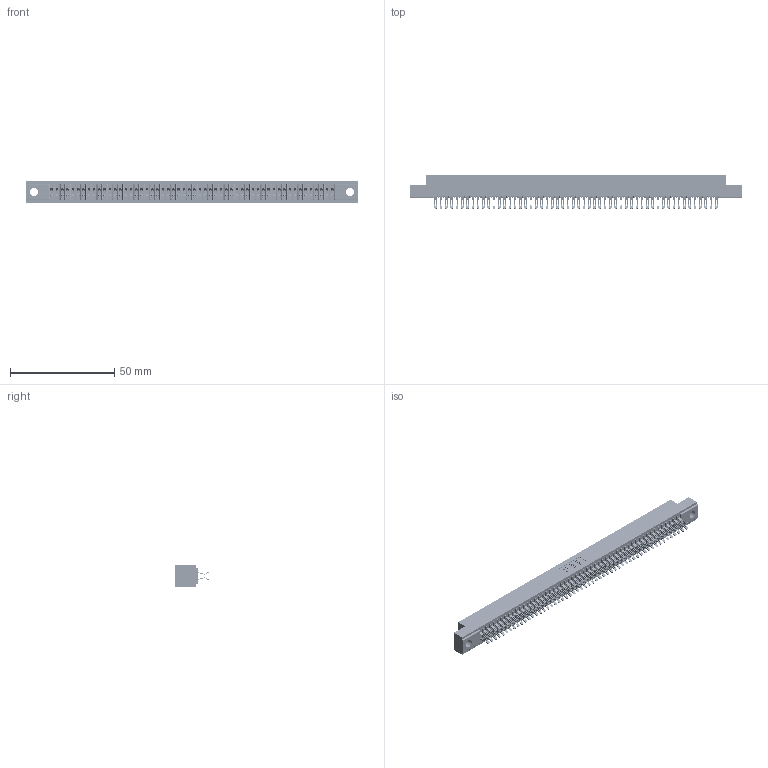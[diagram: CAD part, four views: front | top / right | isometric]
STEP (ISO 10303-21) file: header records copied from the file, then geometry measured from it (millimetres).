
FILE_DESCRIPTION (( 'STEP AP203' ), '1' );
FILE_NAME ('341-108-555-204.STEP', '2018-08-08T12:24:53', ( '' ), ( '' ), 'SwSTEP 2.0', 'SolidWorks 2016', '' );
FILE_SCHEMA (( 'CONFIG_CONTROL_DESIGN' ));
Length unit declared in the file: inch
Products named in the file (3): 341 Part_.156 (3.96) Dia Mounting Holes; 341-292-001_341-292-155; 341-108-555-204
Assembly tree (109 placements, depth 2):
  341-108-555-204
    341 Part_.156 (3.96) Dia Mounting Holes
    341-292-001_341-292-155  x108
Bounding box: 159.38 x 16.31 x 10.16 mm (x, y, z)
Volume: 11811.7 mm3; surface area: 22113.9 mm2
Topology: 109 solids, 109 shells, 8554 faces, 25570 edges, 16646 vertices
Faces by surface type: plane 4618, cylinder 3720, sphere 110, torus 106
Entity records: 64641 total; most frequent: CARTESIAN_POINT 10766, ORIENTED_EDGE 10688, DIRECTION 10422, EDGE_CURVE 5344, LINE 4322, VECTOR 4322, VERTEX_POINT 3378, AXIS2_PLACEMENT_3D 3050
